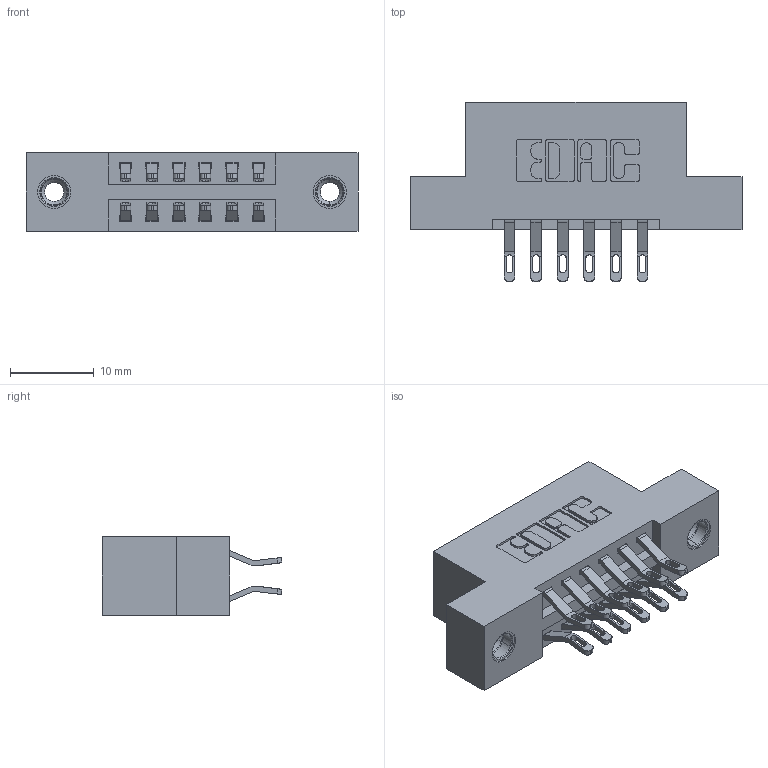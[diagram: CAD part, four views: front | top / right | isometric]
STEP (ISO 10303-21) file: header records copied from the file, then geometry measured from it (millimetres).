
FILE_DESCRIPTION (( 'STEP AP203' ), '1' );
FILE_NAME ('396-012-555-208.STEP', '2019-10-29T19:37:15', ( '' ), ( '' ), 'SwSTEP 2.0', 'SolidWorks 2016', '' );
FILE_SCHEMA (( 'CONFIG_CONTROL_DESIGN' ));
Length unit declared in the file: inch
Products named in the file (4): 346 Part_Flush Mounting Lugs - 0.156 Dia-TI; 345-250-001_345-250-003-102; 345-292-001_555 Tail; 396-012-555-208
Assembly tree (15 placements, depth 2):
  396-012-555-208
    346 Part_Flush Mounting Lugs - 0.156 Dia-TI
    345-292-001_555 Tail  x12
    345-250-001_345-250-003-102  x2
Bounding box: 39.62 x 21.46 x 9.4 mm (x, y, z)
Volume: 3612.5 mm3; surface area: 4543.9 mm2
Topology: 15 solids, 15 shells, 878 faces, 2661 edges, 1766 vertices
Faces by surface type: plane 504, cylinder 358, cone 12, torus 4
Entity records: 10274 total; most frequent: CARTESIAN_POINT 1761, ORIENTED_EDGE 1658, DIRECTION 1599, EDGE_CURVE 829, LINE 633, VECTOR 633, VERTEX_POINT 548, AXIS2_PLACEMENT_3D 483
